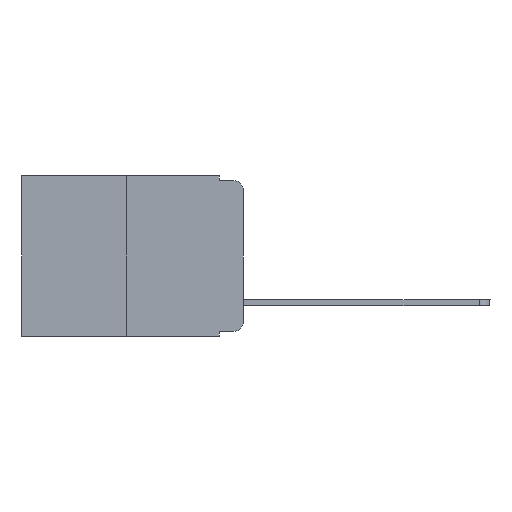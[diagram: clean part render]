
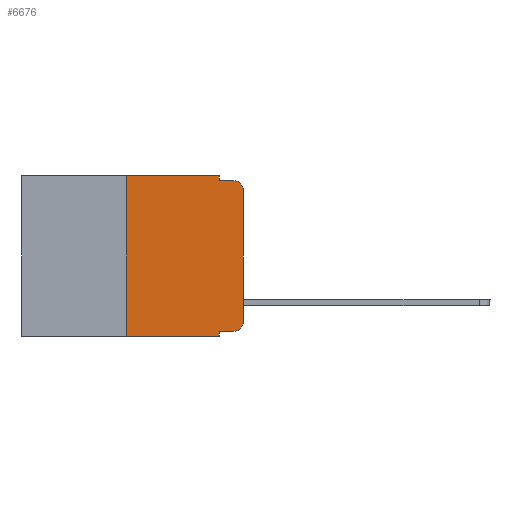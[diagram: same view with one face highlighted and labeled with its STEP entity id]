
A CAD part, left-side view. The second image highlights one B-rep face of the part: STEP entity #6676.
In plain terms, the highlighted planar face has unit normal (-1, 0, 0).
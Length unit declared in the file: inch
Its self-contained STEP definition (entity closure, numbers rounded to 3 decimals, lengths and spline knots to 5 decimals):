
#42 = ORIENTED_EDGE ( 'NONE', *, *, #5920, .F. ) ;
#299 = VECTOR ( 'NONE', #11282, 39.37008 ) ;
#308 = DIRECTION ( 'NONE',  ( 0., 0., -1. ) ) ;
#339 = DIRECTION ( 'NONE',  ( 0., 0., -1. ) ) ;
#547 = CARTESIAN_POINT ( 'NONE',  ( 0., 0.473, 0. ) ) ;
#961 = CARTESIAN_POINT ( 'NONE',  ( 0., 0.25, 0. ) ) ;
#1614 = CARTESIAN_POINT ( 'NONE',  ( 0., 0., -0.313 ) ) ;
#1653 = LINE ( 'NONE', #1692, #15565 ) ;
#1692 = CARTESIAN_POINT ( 'NONE',  ( 0., 0.051, -0.01 ) ) ;
#1960 = AXIS2_PLACEMENT_3D ( 'NONE', #9529, #5904, #308 ) ;
#2119 = ORIENTED_EDGE ( 'NONE', *, *, #13738, .T. ) ;
#2200 = PLANE ( 'NONE',  #1960 ) ;
#2999 = EDGE_CURVE ( 'NONE', #7786, #11496, #8044, .T. ) ;
#3741 = CARTESIAN_POINT ( 'NONE',  ( 0., 0.051, 0. ) ) ;
#4126 = ORIENTED_EDGE ( 'NONE', *, *, #17915, .T. ) ;
#4458 = DIRECTION ( 'NONE',  ( 0., -1., 0. ) ) ;
#4614 = EDGE_CURVE ( 'NONE', #6140, #10125, #21586, .T. ) ;
#4837 = ORIENTED_EDGE ( 'NONE', *, *, #4614, .F. ) ;
#5904 = DIRECTION ( 'NONE',  ( 1., 0., 0. ) ) ;
#5920 = EDGE_CURVE ( 'NONE', #14859, #11496, #1653, .T. ) ;
#6124 = EDGE_CURVE ( 'NONE', #11075, #14859, #7875, .T. ) ;
#6140 = VERTEX_POINT ( 'NONE', #13027 ) ;
#6222 = LINE ( 'NONE', #9740, #299 ) ;
#6378 = DIRECTION ( 'NONE',  ( -1., 0., 0. ) ) ;
#6642 = DIRECTION ( 'NONE',  ( 0., 0., -1. ) ) ;
#6676 = ADVANCED_FACE ( 'NONE', ( #18082 ), #2200, .F. ) ;
#7291 = VERTEX_POINT ( 'NONE', #12826 ) ;
#7708 = CARTESIAN_POINT ( 'NONE',  ( 0., 0.25, 0. ) ) ;
#7786 = VERTEX_POINT ( 'NONE', #10910 ) ;
#7875 = LINE ( 'NONE', #3741, #15832 ) ;
#7885 = DIRECTION ( 'NONE',  ( 0., 0., 1. ) ) ;
#8044 = CIRCLE ( 'NONE', #20441, 0.02 ) ;
#8275 = LINE ( 'NONE', #547, #10569 ) ;
#8627 = VECTOR ( 'NONE', #4458, 39.37008 ) ;
#9485 = AXIS2_PLACEMENT_3D ( 'NONE', #17277, #6378, #13710 ) ;
#9529 = CARTESIAN_POINT ( 'NONE',  ( 0., 0.473, 0. ) ) ;
#9534 = DIRECTION ( 'NONE',  ( 0., -1., 0. ) ) ;
#9568 = CARTESIAN_POINT ( 'NONE',  ( 0., 0.051, -0.333 ) ) ;
#9740 = CARTESIAN_POINT ( 'NONE',  ( 0., 0.473, -0.343 ) ) ;
#9940 = CIRCLE ( 'NONE', #9485, 0.02 ) ;
#10125 = VERTEX_POINT ( 'NONE', #961 ) ;
#10245 = EDGE_CURVE ( 'NONE', #12531, #13066, #12402, .T. ) ;
#10548 = VECTOR ( 'NONE', #22309, 39.37008 ) ;
#10569 = VECTOR ( 'NONE', #9534, 39.37008 ) ;
#10755 = DIRECTION ( 'NONE',  ( 0., -1., 0. ) ) ;
#10819 = VECTOR ( 'NONE', #7885, 39.37008 ) ;
#10838 = VERTEX_POINT ( 'NONE', #1614 ) ;
#10910 = CARTESIAN_POINT ( 'NONE',  ( 0., 0., -0.03 ) ) ;
#11075 = VERTEX_POINT ( 'NONE', #16430 ) ;
#11282 = DIRECTION ( 'NONE',  ( 0., -1., 0. ) ) ;
#11496 = VERTEX_POINT ( 'NONE', #20973 ) ;
#11892 = DIRECTION ( 'NONE',  ( 0., 0., -1. ) ) ;
#11974 = EDGE_CURVE ( 'NONE', #12531, #7291, #13428, .T. ) ;
#12088 = CARTESIAN_POINT ( 'NONE',  ( 0., 0.051, -0.333 ) ) ;
#12402 = LINE ( 'NONE', #15649, #22303 ) ;
#12531 = VERTEX_POINT ( 'NONE', #12088 ) ;
#12682 = ORIENTED_EDGE ( 'NONE', *, *, #10245, .F. ) ;
#12826 = CARTESIAN_POINT ( 'NONE',  ( 0., 0.02, -0.333 ) ) ;
#12834 = EDGE_CURVE ( 'NONE', #10125, #11075, #8275, .T. ) ;
#13012 = CARTESIAN_POINT ( 'NONE',  ( 0., 0.051, -0.01 ) ) ;
#13027 = CARTESIAN_POINT ( 'NONE',  ( 0., 0.25, -0.343 ) ) ;
#13066 = VERTEX_POINT ( 'NONE', #15344 ) ;
#13397 = CARTESIAN_POINT ( 'NONE',  ( 0., 0.02, -0.03 ) ) ;
#13428 = LINE ( 'NONE', #9568, #8627 ) ;
#13498 = ORIENTED_EDGE ( 'NONE', *, *, #2999, .T. ) ;
#13710 = DIRECTION ( 'NONE',  ( 0., 0., -1. ) ) ;
#13738 = EDGE_CURVE ( 'NONE', #7291, #10838, #9940, .T. ) ;
#13780 = EDGE_LOOP ( 'NONE', ( #4126, #13498, #42, #15210, #23418, #4837, #18418, #12682, #14084, #2119 ) ) ;
#14084 = ORIENTED_EDGE ( 'NONE', *, *, #11974, .T. ) ;
#14859 = VERTEX_POINT ( 'NONE', #13012 ) ;
#15210 = ORIENTED_EDGE ( 'NONE', *, *, #6124, .F. ) ;
#15344 = CARTESIAN_POINT ( 'NONE',  ( 0., 0.051, -0.343 ) ) ;
#15565 = VECTOR ( 'NONE', #10755, 39.37008 ) ;
#15649 = CARTESIAN_POINT ( 'NONE',  ( 0., 0.051, 0. ) ) ;
#15832 = VECTOR ( 'NONE', #339, 39.37008 ) ;
#16430 = CARTESIAN_POINT ( 'NONE',  ( 0., 0.051, 0. ) ) ;
#16930 = CARTESIAN_POINT ( 'NONE',  ( 0., 0., 0. ) ) ;
#17277 = CARTESIAN_POINT ( 'NONE',  ( 0., 0.02, -0.313 ) ) ;
#17915 = EDGE_CURVE ( 'NONE', #10838, #7786, #23292, .T. ) ;
#18031 = EDGE_CURVE ( 'NONE', #6140, #13066, #6222, .T. ) ;
#18082 = FACE_OUTER_BOUND ( 'NONE', #13780, .T. ) ;
#18418 = ORIENTED_EDGE ( 'NONE', *, *, #18031, .T. ) ;
#20441 = AXIS2_PLACEMENT_3D ( 'NONE', #13397, #22588, #11892 ) ;
#20973 = CARTESIAN_POINT ( 'NONE',  ( 0., 0.02, -0.01 ) ) ;
#21586 = LINE ( 'NONE', #7708, #10548 ) ;
#22303 = VECTOR ( 'NONE', #6642, 39.37008 ) ;
#22309 = DIRECTION ( 'NONE',  ( 0., 0., 1. ) ) ;
#22588 = DIRECTION ( 'NONE',  ( -1., 0., 0. ) ) ;
#23292 = LINE ( 'NONE', #16930, #10819 ) ;
#23418 = ORIENTED_EDGE ( 'NONE', *, *, #12834, .F. ) ;
